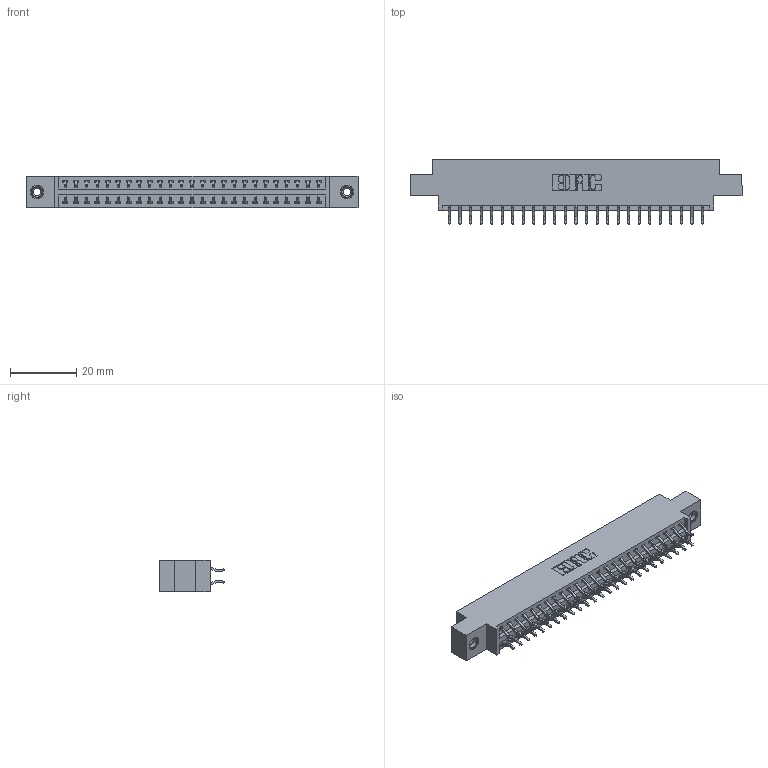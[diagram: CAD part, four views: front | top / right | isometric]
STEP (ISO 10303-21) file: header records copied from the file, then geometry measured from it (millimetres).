
FILE_DESCRIPTION (( 'STEP AP203' ), '1' );
FILE_NAME ('346-050-556-808.STEP', '2018-08-27T22:44:58', ( '' ), ( '' ), 'SwSTEP 2.0', 'SolidWorks 2016', '' );
FILE_SCHEMA (( 'CONFIG_CONTROL_DESIGN' ));
Length unit declared in the file: inch
Products named in the file (4): 346-050-556-808; 346 Part_0.170 Offset - 0.156 Dia-TI; 345-292-001_556 Tail; 345-250-001_345-250-003-102
Assembly tree (53 placements, depth 2):
  346-050-556-808
    346 Part_0.170 Offset - 0.156 Dia-TI
    345-292-001_556 Tail  x50
    345-250-001_345-250-003-102  x2
Bounding box: 99.95 x 19.57 x 9.4 mm (x, y, z)
Volume: 9451.1 mm3; surface area: 12877.2 mm2
Topology: 53 solids, 53 shells, 3086 faces, 9127 edges, 6010 vertices
Faces by surface type: plane 2062, cylinder 1008, cone 12, torus 4
Entity records: 20142 total; most frequent: CARTESIAN_POINT 3343, ORIENTED_EDGE 3258, DIRECTION 3011, EDGE_CURVE 1629, LINE 1369, VECTOR 1369, VERTEX_POINT 1080, AXIS2_PLACEMENT_3D 821
